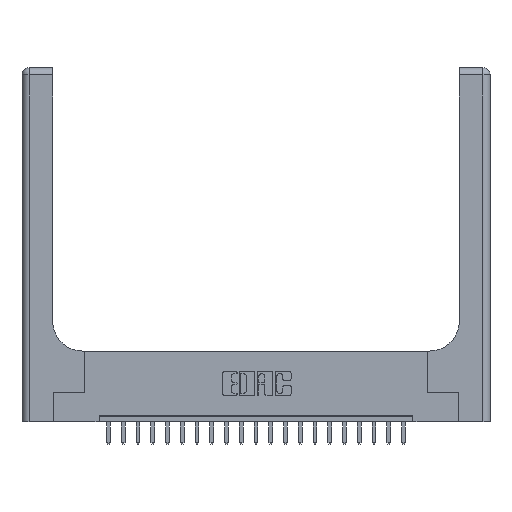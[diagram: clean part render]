
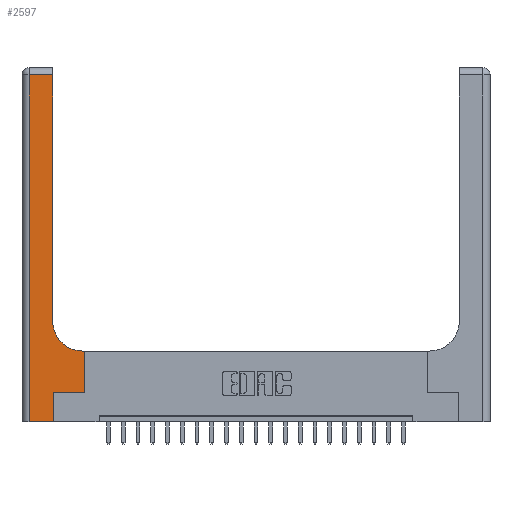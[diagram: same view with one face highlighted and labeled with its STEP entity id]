
A CAD part, top view. The second image highlights one B-rep face of the part: STEP entity #2597.
In plain terms, the highlighted planar face has unit normal (0, 0, 1).
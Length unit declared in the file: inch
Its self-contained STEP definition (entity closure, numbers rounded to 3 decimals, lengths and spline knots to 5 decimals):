
#180 = CARTESIAN_POINT ( 'NONE',  ( 0.26, 3., 0.37 ) ) ;
#398 = LINE ( 'NONE', #180, #3429 ) ;
#588 = CIRCLE ( 'NONE', #16304, 0.25 ) ;
#661 = EDGE_CURVE ( 'NONE', #13657, #3238, #3245, .T. ) ;
#678 = LINE ( 'NONE', #20347, #11111 ) ;
#797 = CARTESIAN_POINT ( 'NONE',  ( 0.26, 2.94, 0.37 ) ) ;
#915 = CARTESIAN_POINT ( 'NONE',  ( 0.528, 0.6, 0.37 ) ) ;
#1193 = CARTESIAN_POINT ( 'NONE',  ( 0.06, 3., 0.37 ) ) ;
#1831 = VERTEX_POINT ( 'NONE', #15753 ) ;
#2138 = DIRECTION ( 'NONE',  ( 0., 1., 0. ) ) ;
#2160 = LINE ( 'NONE', #17023, #15617 ) ;
#2518 = VECTOR ( 'NONE', #11653, 39.37008 ) ;
#2597 = ADVANCED_FACE ( 'NONE', ( #15333 ), #18933, .F. ) ;
#2902 = EDGE_LOOP ( 'NONE', ( #13326, #15593, #4880, #15648, #10793, #5218, #4324, #10934, #10350 ) ) ;
#2954 = CARTESIAN_POINT ( 'NONE',  ( 0.265, 0.25, 0.37 ) ) ;
#3238 = VERTEX_POINT ( 'NONE', #12914 ) ;
#3245 = LINE ( 'NONE', #1193, #2518 ) ;
#3273 = DIRECTION ( 'NONE',  ( 1., 0., 0. ) ) ;
#3429 = VECTOR ( 'NONE', #2138, 39.37008 ) ;
#4095 = VECTOR ( 'NONE', #20060, 39.37008 ) ;
#4324 = ORIENTED_EDGE ( 'NONE', *, *, #4688, .T. ) ;
#4476 = EDGE_CURVE ( 'NONE', #12699, #9837, #16377, .T. ) ;
#4688 = EDGE_CURVE ( 'NONE', #9837, #6262, #2160, .T. ) ;
#4880 = ORIENTED_EDGE ( 'NONE', *, *, #661, .T. ) ;
#5055 = EDGE_CURVE ( 'NONE', #17704, #17883, #398, .T. ) ;
#5218 = ORIENTED_EDGE ( 'NONE', *, *, #4476, .T. ) ;
#5659 = CARTESIAN_POINT ( 'NONE',  ( 0.265, 0., 0.37 ) ) ;
#6262 = VERTEX_POINT ( 'NONE', #915 ) ;
#6870 = DIRECTION ( 'NONE',  ( 0., 1., 0. ) ) ;
#7168 = DIRECTION ( 'NONE',  ( 0., 1., 0. ) ) ;
#8972 = DIRECTION ( 'NONE',  ( -1., 0., 0. ) ) ;
#9025 = CARTESIAN_POINT ( 'NONE',  ( 0.265, 0.25, 0.37 ) ) ;
#9045 = VECTOR ( 'NONE', #7168, 39.37008 ) ;
#9837 = VERTEX_POINT ( 'NONE', #10250 ) ;
#9905 = LINE ( 'NONE', #11562, #4095 ) ;
#10250 = CARTESIAN_POINT ( 'NONE',  ( 0.528, 0.25, 0.37 ) ) ;
#10350 = ORIENTED_EDGE ( 'NONE', *, *, #15535, .T. ) ;
#10738 = DIRECTION ( 'NONE',  ( 0., 0., -1. ) ) ;
#10793 = ORIENTED_EDGE ( 'NONE', *, *, #20117, .T. ) ;
#10934 = ORIENTED_EDGE ( 'NONE', *, *, #15821, .T. ) ;
#11111 = VECTOR ( 'NONE', #8972, 39.37008 ) ;
#11562 = CARTESIAN_POINT ( 'NONE',  ( 0.26, 0.6, 0.37 ) ) ;
#11593 = CARTESIAN_POINT ( 'NONE',  ( 0., 0., 0.37 ) ) ;
#11653 = DIRECTION ( 'NONE',  ( 0., -1., 0. ) ) ;
#12630 = EDGE_CURVE ( 'NONE', #3238, #17039, #21531, .T. ) ;
#12699 = VERTEX_POINT ( 'NONE', #9025 ) ;
#12914 = CARTESIAN_POINT ( 'NONE',  ( 0.06, 0., 0.37 ) ) ;
#13234 = CARTESIAN_POINT ( 'NONE',  ( 0.265, 0., 0.37 ) ) ;
#13326 = ORIENTED_EDGE ( 'NONE', *, *, #5055, .T. ) ;
#13456 = EDGE_CURVE ( 'NONE', #17883, #13657, #678, .T. ) ;
#13477 = DIRECTION ( 'NONE',  ( 0., 0., -1. ) ) ;
#13601 = DIRECTION ( 'NONE',  ( -1., 0., 0. ) ) ;
#13657 = VERTEX_POINT ( 'NONE', #21605 ) ;
#15333 = FACE_OUTER_BOUND ( 'NONE', #2902, .T. ) ;
#15340 = CARTESIAN_POINT ( 'NONE',  ( 0.26, 0.85, 0.37 ) ) ;
#15475 = LINE ( 'NONE', #5659, #9045 ) ;
#15535 = EDGE_CURVE ( 'NONE', #1831, #17704, #588, .T. ) ;
#15593 = ORIENTED_EDGE ( 'NONE', *, *, #13456, .T. ) ;
#15617 = VECTOR ( 'NONE', #6870, 39.37008 ) ;
#15648 = ORIENTED_EDGE ( 'NONE', *, *, #12630, .T. ) ;
#15731 = DIRECTION ( 'NONE',  ( 1., 0., 0. ) ) ;
#15753 = CARTESIAN_POINT ( 'NONE',  ( 0.51, 0.6, 0.37 ) ) ;
#15821 = EDGE_CURVE ( 'NONE', #6262, #1831, #9905, .T. ) ;
#16304 = AXIS2_PLACEMENT_3D ( 'NONE', #17354, #13477, #15731 ) ;
#16377 = LINE ( 'NONE', #2954, #18753 ) ;
#17023 = CARTESIAN_POINT ( 'NONE',  ( 0.528, 0.25, 0.37 ) ) ;
#17039 = VERTEX_POINT ( 'NONE', #13234 ) ;
#17354 = CARTESIAN_POINT ( 'NONE',  ( 0.51, 0.85, 0.37 ) ) ;
#17704 = VERTEX_POINT ( 'NONE', #15340 ) ;
#17883 = VERTEX_POINT ( 'NONE', #797 ) ;
#18242 = DIRECTION ( 'NONE',  ( 1., 0., 0. ) ) ;
#18703 = CARTESIAN_POINT ( 'NONE',  ( 0., 3., 0.37 ) ) ;
#18753 = VECTOR ( 'NONE', #3273, 39.37008 ) ;
#18933 = PLANE ( 'NONE',  #19699 ) ;
#19699 = AXIS2_PLACEMENT_3D ( 'NONE', #18703, #10738, #13601 ) ;
#20060 = DIRECTION ( 'NONE',  ( -1., 0., 0. ) ) ;
#20117 = EDGE_CURVE ( 'NONE', #17039, #12699, #15475, .T. ) ;
#20347 = CARTESIAN_POINT ( 'NONE',  ( 0., 2.94, 0.37 ) ) ;
#21519 = VECTOR ( 'NONE', #18242, 39.37008 ) ;
#21531 = LINE ( 'NONE', #11593, #21519 ) ;
#21605 = CARTESIAN_POINT ( 'NONE',  ( 0.06, 2.94, 0.37 ) ) ;
